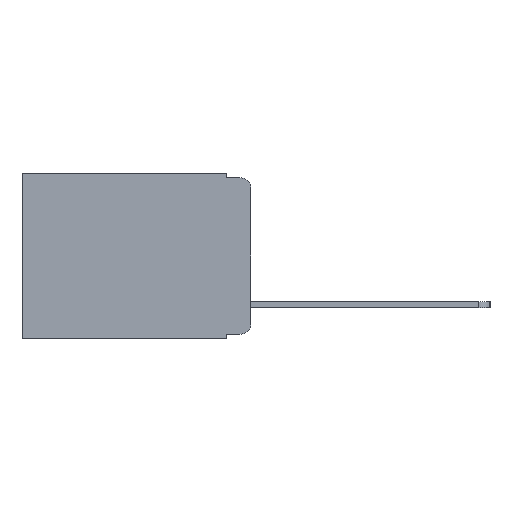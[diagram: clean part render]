
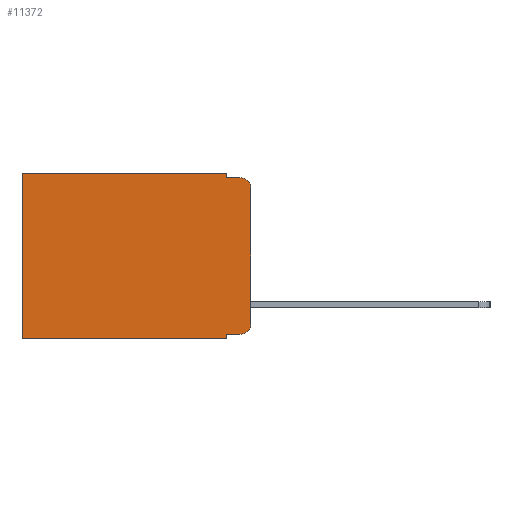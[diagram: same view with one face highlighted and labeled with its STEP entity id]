
A CAD part, left-side view. The second image highlights one B-rep face of the part: STEP entity #11372.
In plain terms, the highlighted planar face has unit normal (-1, 0, 0).
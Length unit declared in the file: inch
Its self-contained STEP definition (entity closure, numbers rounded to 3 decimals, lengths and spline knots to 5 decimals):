
#323 = DIRECTION ( 'NONE',  ( -1., 0., 0. ) ) ;
#436 = CARTESIAN_POINT ( 'NONE',  ( 0.298, 0.051, -0.01 ) ) ;
#585 = EDGE_CURVE ( 'NONE', #2185, #4999, #7703, .T. ) ;
#661 = VERTEX_POINT ( 'NONE', #2244 ) ;
#664 = EDGE_CURVE ( 'NONE', #2185, #5851, #1434, .T. ) ;
#744 = EDGE_CURVE ( 'NONE', #16797, #5851, #8457, .T. ) ;
#781 = EDGE_CURVE ( 'NONE', #9038, #16797, #7439, .T. ) ;
#818 = EDGE_CURVE ( 'NONE', #7141, #11003, #2289, .T. ) ;
#843 = EDGE_CURVE ( 'NONE', #2512, #11003, #13479, .T. ) ;
#846 = EDGE_CURVE ( 'NONE', #3344, #2512, #19543, .T. ) ;
#874 = EDGE_CURVE ( 'NONE', #3344, #661, #8717, .T. ) ;
#881 = EDGE_CURVE ( 'NONE', #661, #4999, #15799, .T. ) ;
#1395 = DIRECTION ( 'NONE',  ( 0., 0., -1. ) ) ;
#1434 = CIRCLE ( 'NONE', #15585, 0.02 ) ;
#1692 = EDGE_LOOP ( 'NONE', ( #2464, #12146, #7026, #2678, #4239, #9572, #9665, #2696, #4987, #5059 ) ) ;
#1739 = CARTESIAN_POINT ( 'NONE',  ( 0.298, 0.051, -0.343 ) ) ;
#2185 = VERTEX_POINT ( 'NONE', #5600 ) ;
#2244 = CARTESIAN_POINT ( 'NONE',  ( 0.298, 0.02, -0.333 ) ) ;
#2289 = LINE ( 'NONE', #9273, #17332 ) ;
#2464 = ORIENTED_EDGE ( 'NONE', *, *, #585, .F. ) ;
#2512 = VERTEX_POINT ( 'NONE', #1739 ) ;
#2678 = ORIENTED_EDGE ( 'NONE', *, *, #781, .F. ) ;
#2696 = ORIENTED_EDGE ( 'NONE', *, *, #846, .F. ) ;
#2866 = VECTOR ( 'NONE', #13671, 39.37008 ) ;
#3344 = VERTEX_POINT ( 'NONE', #16209 ) ;
#3759 = VECTOR ( 'NONE', #7695, 39.37008 ) ;
#4103 = DIRECTION ( 'NONE',  ( 0., 0., -1. ) ) ;
#4239 = ORIENTED_EDGE ( 'NONE', *, *, #16381, .T. ) ;
#4332 = VECTOR ( 'NONE', #19047, 39.37008 ) ;
#4987 = ORIENTED_EDGE ( 'NONE', *, *, #874, .T. ) ;
#4999 = VERTEX_POINT ( 'NONE', #7290 ) ;
#5059 = ORIENTED_EDGE ( 'NONE', *, *, #881, .T. ) ;
#5241 = DIRECTION ( 'NONE',  ( 0., -1., 0. ) ) ;
#5358 = VECTOR ( 'NONE', #15145, 39.37008 ) ;
#5600 = CARTESIAN_POINT ( 'NONE',  ( 0.298, 0., -0.03 ) ) ;
#5851 = VERTEX_POINT ( 'NONE', #9537 ) ;
#5907 = CARTESIAN_POINT ( 'NONE',  ( 0.298, 0.051, -0.01 ) ) ;
#5972 = FACE_OUTER_BOUND ( 'NONE', #1692, .T. ) ;
#6084 = CARTESIAN_POINT ( 'NONE',  ( 0.298, 0.02, -0.313 ) ) ;
#6341 = CARTESIAN_POINT ( 'NONE',  ( 0.298, 0.051, 0. ) ) ;
#7026 = ORIENTED_EDGE ( 'NONE', *, *, #744, .F. ) ;
#7141 = VERTEX_POINT ( 'NONE', #15617 ) ;
#7290 = CARTESIAN_POINT ( 'NONE',  ( 0.298, 0., -0.313 ) ) ;
#7439 = LINE ( 'NONE', #6341, #2866 ) ;
#7695 = DIRECTION ( 'NONE',  ( 0., -1., 0. ) ) ;
#7703 = LINE ( 'NONE', #17437, #4332 ) ;
#8457 = LINE ( 'NONE', #436, #15577 ) ;
#8717 = LINE ( 'NONE', #14750, #3759 ) ;
#9038 = VERTEX_POINT ( 'NONE', #19109 ) ;
#9273 = CARTESIAN_POINT ( 'NONE',  ( 0.298, 0.473, 0. ) ) ;
#9537 = CARTESIAN_POINT ( 'NONE',  ( 0.298, 0.02, -0.01 ) ) ;
#9572 = ORIENTED_EDGE ( 'NONE', *, *, #818, .T. ) ;
#9637 = AXIS2_PLACEMENT_3D ( 'NONE', #6084, #14692, #1395 ) ;
#9665 = ORIENTED_EDGE ( 'NONE', *, *, #843, .F. ) ;
#11003 = VERTEX_POINT ( 'NONE', #19519 ) ;
#11372 = ADVANCED_FACE ( 'NONE', ( #5972 ), #11671, .F. ) ;
#11646 = DIRECTION ( 'NONE',  ( 0., 0., -1. ) ) ;
#11654 = DIRECTION ( 'NONE',  ( 1., 0., 0. ) ) ;
#11671 = PLANE ( 'NONE',  #17674 ) ;
#12146 = ORIENTED_EDGE ( 'NONE', *, *, #664, .T. ) ;
#12920 = VECTOR ( 'NONE', #13797, 39.37008 ) ;
#13062 = VECTOR ( 'NONE', #16044, 39.37008 ) ;
#13346 = LINE ( 'NONE', #15161, #12920 ) ;
#13479 = LINE ( 'NONE', #18572, #13062 ) ;
#13592 = CARTESIAN_POINT ( 'NONE',  ( 0.298, 0., 0. ) ) ;
#13671 = DIRECTION ( 'NONE',  ( 0., 0., -1. ) ) ;
#13797 = DIRECTION ( 'NONE',  ( 0., 1., 0. ) ) ;
#14692 = DIRECTION ( 'NONE',  ( -1., 0., 0. ) ) ;
#14750 = CARTESIAN_POINT ( 'NONE',  ( 0.298, 0.051, -0.333 ) ) ;
#15145 = DIRECTION ( 'NONE',  ( 0., 0., -1. ) ) ;
#15161 = CARTESIAN_POINT ( 'NONE',  ( 0.298, 0., 0. ) ) ;
#15577 = VECTOR ( 'NONE', #5241, 39.37008 ) ;
#15585 = AXIS2_PLACEMENT_3D ( 'NONE', #18571, #323, #17887 ) ;
#15617 = CARTESIAN_POINT ( 'NONE',  ( 0.298, 0.473, 0. ) ) ;
#15799 = CIRCLE ( 'NONE', #9637, 0.02 ) ;
#15847 = CARTESIAN_POINT ( 'NONE',  ( 0.298, 0.051, 0. ) ) ;
#16044 = DIRECTION ( 'NONE',  ( 0., 1., 0. ) ) ;
#16209 = CARTESIAN_POINT ( 'NONE',  ( 0.298, 0.051, -0.333 ) ) ;
#16381 = EDGE_CURVE ( 'NONE', #9038, #7141, #13346, .T. ) ;
#16797 = VERTEX_POINT ( 'NONE', #5907 ) ;
#17332 = VECTOR ( 'NONE', #4103, 39.37008 ) ;
#17437 = CARTESIAN_POINT ( 'NONE',  ( 0.298, 0., 0. ) ) ;
#17674 = AXIS2_PLACEMENT_3D ( 'NONE', #13592, #11654, #11646 ) ;
#17887 = DIRECTION ( 'NONE',  ( 0., 0., -1. ) ) ;
#18571 = CARTESIAN_POINT ( 'NONE',  ( 0.298, 0.02, -0.03 ) ) ;
#18572 = CARTESIAN_POINT ( 'NONE',  ( 0.298, 0., -0.343 ) ) ;
#19047 = DIRECTION ( 'NONE',  ( 0., 0., -1. ) ) ;
#19109 = CARTESIAN_POINT ( 'NONE',  ( 0.298, 0.051, 0. ) ) ;
#19519 = CARTESIAN_POINT ( 'NONE',  ( 0.298, 0.473, -0.343 ) ) ;
#19543 = LINE ( 'NONE', #15847, #5358 ) ;
